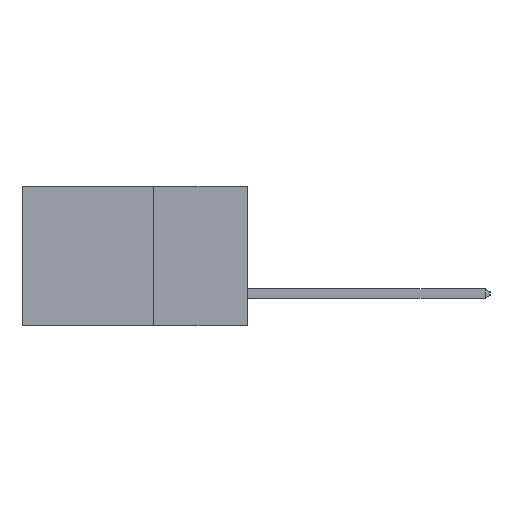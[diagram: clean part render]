
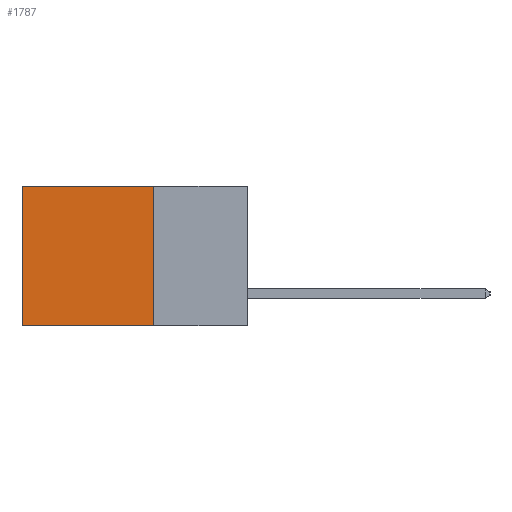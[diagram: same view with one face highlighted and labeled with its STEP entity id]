
A CAD part, left-side view. The second image highlights one B-rep face of the part: STEP entity #1787.
In plain terms, the highlighted planar face has unit normal (-1, 0, 0).
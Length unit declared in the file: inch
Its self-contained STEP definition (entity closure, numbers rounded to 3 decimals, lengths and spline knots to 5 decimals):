
#711 = AXIS2_PLACEMENT_3D ( 'NONE', #10063, #10177, #10889 ) ;
#1061 = CARTESIAN_POINT ( 'NONE',  ( 0.298, 0.6, 0. ) ) ;
#1424 = EDGE_CURVE ( 'NONE', #1522, #9075, #4001, .T. ) ;
#1522 = VERTEX_POINT ( 'NONE', #11786 ) ;
#1787 = ADVANCED_FACE ( 'NONE', ( #5648 ), #8344, .F. ) ;
#1948 = DIRECTION ( 'NONE',  ( 0., 0., -1. ) ) ;
#2530 = VECTOR ( 'NONE', #4249, 39.37008 ) ;
#3528 = VECTOR ( 'NONE', #9183, 39.37008 ) ;
#3651 = VECTOR ( 'NONE', #1948, 39.37008 ) ;
#4001 = LINE ( 'NONE', #7008, #14081 ) ;
#4249 = DIRECTION ( 'NONE',  ( 0., 0., -1. ) ) ;
#5290 = LINE ( 'NONE', #12143, #2530 ) ;
#5648 = FACE_OUTER_BOUND ( 'NONE', #11601, .T. ) ;
#6252 = VERTEX_POINT ( 'NONE', #12413 ) ;
#7008 = CARTESIAN_POINT ( 'NONE',  ( 0.298, 0.25, -0.37 ) ) ;
#7540 = LINE ( 'NONE', #10462, #3528 ) ;
#8192 = CARTESIAN_POINT ( 'NONE',  ( 0.298, 0.6, -0.37 ) ) ;
#8266 = EDGE_CURVE ( 'NONE', #6252, #9553, #7540, .T. ) ;
#8344 = PLANE ( 'NONE',  #711 ) ;
#9075 = VERTEX_POINT ( 'NONE', #8192 ) ;
#9183 = DIRECTION ( 'NONE',  ( 0., 1., 0. ) ) ;
#9553 = VERTEX_POINT ( 'NONE', #1061 ) ;
#9571 = ORIENTED_EDGE ( 'NONE', *, *, #8266, .T. ) ;
#9889 = LINE ( 'NONE', #9970, #3651 ) ;
#9970 = CARTESIAN_POINT ( 'NONE',  ( 0.298, 0.6, 0. ) ) ;
#10063 = CARTESIAN_POINT ( 'NONE',  ( 0.298, 0.25, 0. ) ) ;
#10177 = DIRECTION ( 'NONE',  ( 1., 0., 0. ) ) ;
#10462 = CARTESIAN_POINT ( 'NONE',  ( 0.298, 0.25, 0. ) ) ;
#10865 = ORIENTED_EDGE ( 'NONE', *, *, #14210, .T. ) ;
#10889 = DIRECTION ( 'NONE',  ( 0., 0., -1. ) ) ;
#11601 = EDGE_LOOP ( 'NONE', ( #10865, #16018, #12275, #9571 ) ) ;
#11786 = CARTESIAN_POINT ( 'NONE',  ( 0.298, 0.25, -0.37 ) ) ;
#12143 = CARTESIAN_POINT ( 'NONE',  ( 0.298, 0.25, 0. ) ) ;
#12275 = ORIENTED_EDGE ( 'NONE', *, *, #15308, .F. ) ;
#12413 = CARTESIAN_POINT ( 'NONE',  ( 0.298, 0.25, 0. ) ) ;
#14081 = VECTOR ( 'NONE', #15564, 39.37008 ) ;
#14210 = EDGE_CURVE ( 'NONE', #9553, #9075, #9889, .T. ) ;
#15308 = EDGE_CURVE ( 'NONE', #6252, #1522, #5290, .T. ) ;
#15564 = DIRECTION ( 'NONE',  ( 0., 1., 0. ) ) ;
#16018 = ORIENTED_EDGE ( 'NONE', *, *, #1424, .F. ) ;
